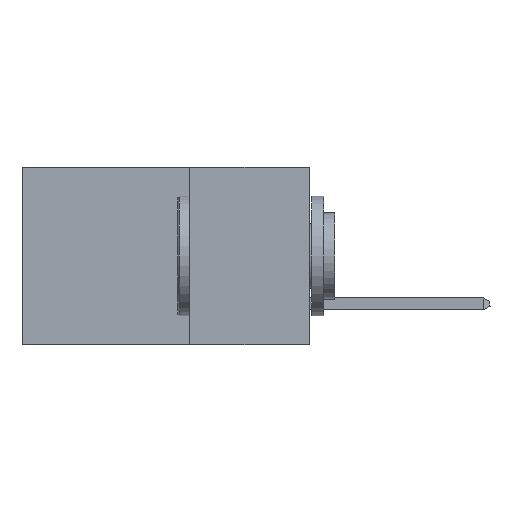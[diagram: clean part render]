
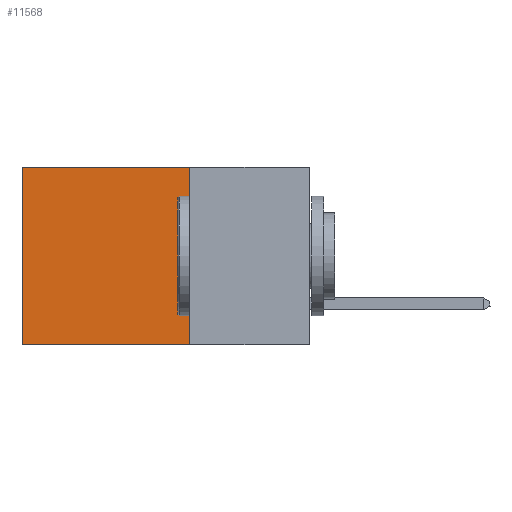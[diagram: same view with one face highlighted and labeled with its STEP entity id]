
A CAD part, left-side view. The second image highlights one B-rep face of the part: STEP entity #11568.
In plain terms, the highlighted planar face has unit normal (-1, 0, 0).
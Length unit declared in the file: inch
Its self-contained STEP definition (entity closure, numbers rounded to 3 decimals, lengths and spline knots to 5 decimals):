
#946 = LINE ( 'NONE', #10375, #4126 ) ;
#1625 = DIRECTION ( 'NONE',  ( 0., 0., -1. ) ) ;
#1664 = AXIS2_PLACEMENT_3D ( 'NONE', #9939, #8952, #2310 ) ;
#2310 = DIRECTION ( 'NONE',  ( 0., 0., -1. ) ) ;
#2388 = VECTOR ( 'NONE', #2919, 39.37008 ) ;
#2919 = DIRECTION ( 'NONE',  ( 0., 1., 0. ) ) ;
#3446 = VERTEX_POINT ( 'NONE', #6069 ) ;
#3626 = FACE_OUTER_BOUND ( 'NONE', #10378, .T. ) ;
#3674 = LINE ( 'NONE', #4769, #9917 ) ;
#3694 = VERTEX_POINT ( 'NONE', #9481 ) ;
#4126 = VECTOR ( 'NONE', #5504, 39.37008 ) ;
#4152 = DIRECTION ( 'NONE',  ( 0., 0., -1. ) ) ;
#4769 = CARTESIAN_POINT ( 'NONE',  ( 0.2875, 0.6, 0. ) ) ;
#4842 = EDGE_CURVE ( 'NONE', #9403, #12024, #12029, .T. ) ;
#4990 = ORIENTED_EDGE ( 'NONE', *, *, #10783, .T. ) ;
#5504 = DIRECTION ( 'NONE',  ( 0., 1., 0. ) ) ;
#5617 = EDGE_CURVE ( 'NONE', #3446, #3694, #3674, .T. ) ;
#5750 = CARTESIAN_POINT ( 'NONE',  ( 0.2875, 0.25, -0.37 ) ) ;
#5964 = CARTESIAN_POINT ( 'NONE',  ( 0.2875, 0.25, 0. ) ) ;
#6069 = CARTESIAN_POINT ( 'NONE',  ( 0.2875, 0.6, 0. ) ) ;
#7766 = EDGE_CURVE ( 'NONE', #12024, #3694, #10126, .T. ) ;
#7914 = ORIENTED_EDGE ( 'NONE', *, *, #4842, .F. ) ;
#7958 = VECTOR ( 'NONE', #4152, 39.37008 ) ;
#8121 = CARTESIAN_POINT ( 'NONE',  ( 0.2875, 0.25, 0. ) ) ;
#8952 = DIRECTION ( 'NONE',  ( 1., 0., 0. ) ) ;
#9403 = VERTEX_POINT ( 'NONE', #8121 ) ;
#9481 = CARTESIAN_POINT ( 'NONE',  ( 0.2875, 0.6, -0.37 ) ) ;
#9779 = CARTESIAN_POINT ( 'NONE',  ( 0.2875, 0.25, -0.37 ) ) ;
#9917 = VECTOR ( 'NONE', #1625, 39.37008 ) ;
#9939 = CARTESIAN_POINT ( 'NONE',  ( 0.2875, 0.25, 0. ) ) ;
#10126 = LINE ( 'NONE', #9779, #2388 ) ;
#10375 = CARTESIAN_POINT ( 'NONE',  ( 0.2875, 0.25, 0. ) ) ;
#10378 = EDGE_LOOP ( 'NONE', ( #12431, #11247, #7914, #4990 ) ) ;
#10783 = EDGE_CURVE ( 'NONE', #9403, #3446, #946, .T. ) ;
#10923 = PLANE ( 'NONE',  #1664 ) ;
#11247 = ORIENTED_EDGE ( 'NONE', *, *, #7766, .F. ) ;
#11568 = ADVANCED_FACE ( 'NONE', ( #3626 ), #10923, .F. ) ;
#12024 = VERTEX_POINT ( 'NONE', #5750 ) ;
#12029 = LINE ( 'NONE', #5964, #7958 ) ;
#12431 = ORIENTED_EDGE ( 'NONE', *, *, #5617, .T. ) ;
